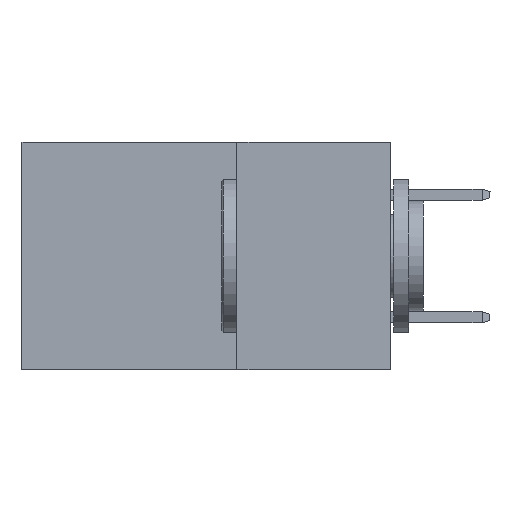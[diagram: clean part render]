
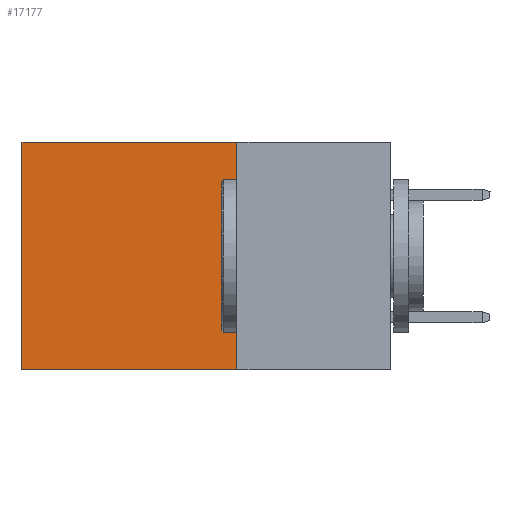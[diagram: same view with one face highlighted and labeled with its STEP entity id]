
A CAD part, left-side view. The second image highlights one B-rep face of the part: STEP entity #17177.
In plain terms, the highlighted planar face has unit normal (-1, 0, 0).
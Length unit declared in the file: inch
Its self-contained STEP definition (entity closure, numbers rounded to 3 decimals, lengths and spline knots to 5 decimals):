
#242 = CARTESIAN_POINT ( 'NONE',  ( 0.2875, 0.25, 0. ) ) ;
#317 = DIRECTION ( 'NONE',  ( 0., 1., 0. ) ) ;
#576 = VERTEX_POINT ( 'NONE', #1710 ) ;
#877 = EDGE_CURVE ( 'NONE', #5101, #576, #14504, .T. ) ;
#1685 = VECTOR ( 'NONE', #5792, 39.37008 ) ;
#1710 = CARTESIAN_POINT ( 'NONE',  ( 0.2875, 0.6, 0. ) ) ;
#2071 = DIRECTION ( 'NONE',  ( 1., 0., 0. ) ) ;
#2076 = LINE ( 'NONE', #18344, #15905 ) ;
#2166 = ORIENTED_EDGE ( 'NONE', *, *, #877, .T. ) ;
#2261 = LINE ( 'NONE', #9360, #1685 ) ;
#2368 = ORIENTED_EDGE ( 'NONE', *, *, #23118, .T. ) ;
#2566 = CARTESIAN_POINT ( 'NONE',  ( 0.2875, 0.25, 0. ) ) ;
#5101 = VERTEX_POINT ( 'NONE', #2566 ) ;
#5792 = DIRECTION ( 'NONE',  ( 0., 0., -1. ) ) ;
#5853 = EDGE_CURVE ( 'NONE', #5101, #20137, #8704, .T. ) ;
#6598 = CARTESIAN_POINT ( 'NONE',  ( 0.2875, 0.6, -0.37 ) ) ;
#8704 = LINE ( 'NONE', #12463, #21841 ) ;
#9356 = DIRECTION ( 'NONE',  ( 0., 1., 0. ) ) ;
#9360 = CARTESIAN_POINT ( 'NONE',  ( 0.2875, 0.6, 0. ) ) ;
#9690 = VECTOR ( 'NONE', #317, 39.37008 ) ;
#11085 = PLANE ( 'NONE',  #17411 ) ;
#12463 = CARTESIAN_POINT ( 'NONE',  ( 0.2875, 0.25, 0. ) ) ;
#12877 = CARTESIAN_POINT ( 'NONE',  ( 0.2875, 0.25, 0. ) ) ;
#14257 = DIRECTION ( 'NONE',  ( 0., 0., -1. ) ) ;
#14504 = LINE ( 'NONE', #242, #9690 ) ;
#14683 = DIRECTION ( 'NONE',  ( 0., 0., -1. ) ) ;
#15066 = EDGE_LOOP ( 'NONE', ( #2368, #15877, #18175, #2166 ) ) ;
#15877 = ORIENTED_EDGE ( 'NONE', *, *, #21270, .F. ) ;
#15905 = VECTOR ( 'NONE', #9356, 39.37008 ) ;
#17177 = ADVANCED_FACE ( 'NONE', ( #21803 ), #11085, .F. ) ;
#17411 = AXIS2_PLACEMENT_3D ( 'NONE', #12877, #2071, #14683 ) ;
#17752 = CARTESIAN_POINT ( 'NONE',  ( 0.2875, 0.25, -0.37 ) ) ;
#18175 = ORIENTED_EDGE ( 'NONE', *, *, #5853, .F. ) ;
#18344 = CARTESIAN_POINT ( 'NONE',  ( 0.2875, 0.25, -0.37 ) ) ;
#20137 = VERTEX_POINT ( 'NONE', #17752 ) ;
#21270 = EDGE_CURVE ( 'NONE', #20137, #21572, #2076, .T. ) ;
#21572 = VERTEX_POINT ( 'NONE', #6598 ) ;
#21803 = FACE_OUTER_BOUND ( 'NONE', #15066, .T. ) ;
#21841 = VECTOR ( 'NONE', #14257, 39.37008 ) ;
#23118 = EDGE_CURVE ( 'NONE', #576, #21572, #2261, .T. ) ;
